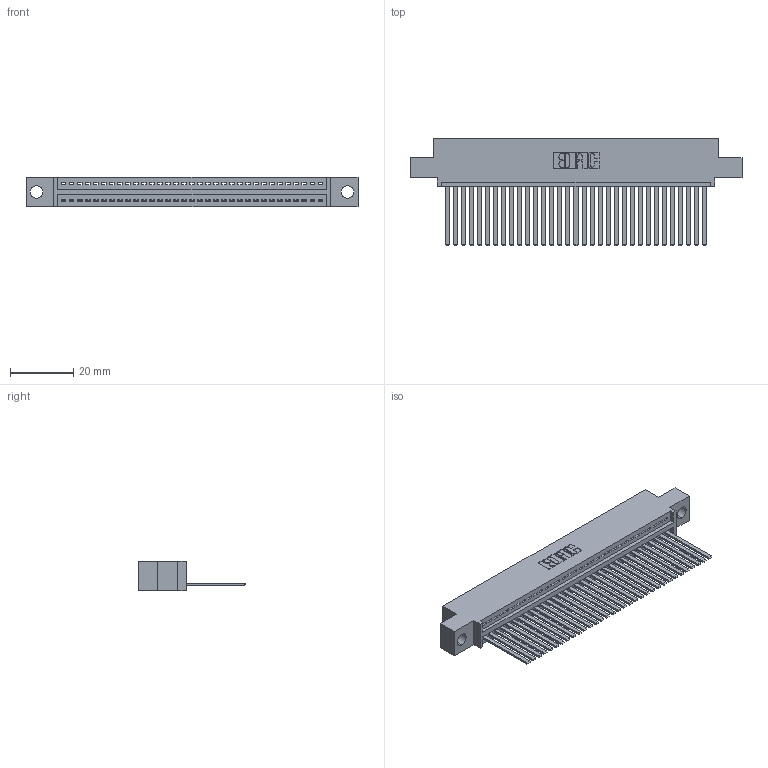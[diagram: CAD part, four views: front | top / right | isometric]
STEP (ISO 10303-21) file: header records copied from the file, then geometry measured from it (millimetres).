
FILE_DESCRIPTION (( 'STEP AP203' ), '1' );
FILE_NAME ('395-033-544-404.STEP', '2018-11-13T03:58:15', ( '' ), ( '' ), 'SwSTEP 2.0', 'SolidWorks 2016', '' );
FILE_SCHEMA (( 'CONFIG_CONTROL_DESIGN' ));
Length unit declared in the file: inch
Products named in the file (3): 395-033-544-404; 345-292-001_345-293-144; 345 Part_0.110 Offset - 0.156 Dia-TH
Assembly tree (34 placements, depth 2):
  395-033-544-404
    345 Part_0.110 Offset - 0.156 Dia-TH
    345-292-001_345-293-144  x33
Bounding box: 105.03 x 33.96 x 9.4 mm (x, y, z)
Volume: 10123 mm3; surface area: 14368.2 mm2
Topology: 34 solids, 34 shells, 1846 faces, 5567 edges, 3666 vertices
Faces by surface type: plane 1272, cylinder 574
Entity records: 25999 total; most frequent: CARTESIAN_POINT 4511, ORIENTED_EDGE 4478, DIRECTION 3949, EDGE_CURVE 2239, LINE 1979, VECTOR 1979, VERTEX_POINT 1490, AXIS2_PLACEMENT_3D 985
